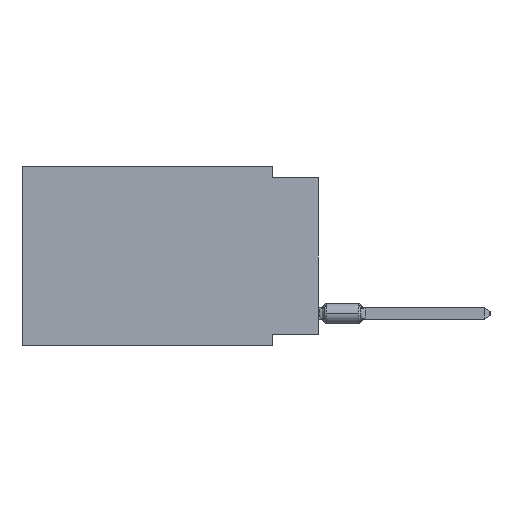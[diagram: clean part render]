
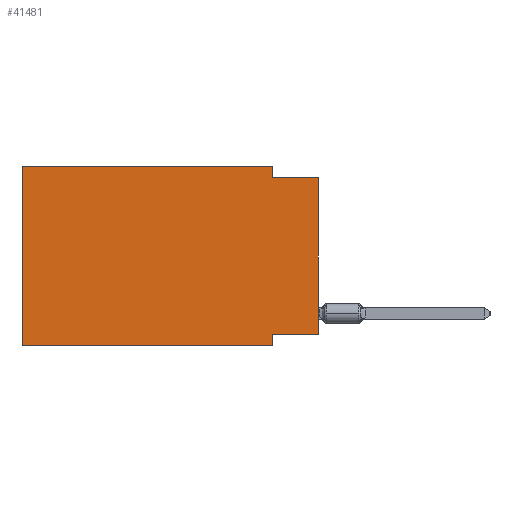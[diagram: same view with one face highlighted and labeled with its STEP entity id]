
A CAD part, left-side view. The second image highlights one B-rep face of the part: STEP entity #41481.
In plain terms, the highlighted planar face has unit normal (-1, 0, 0).
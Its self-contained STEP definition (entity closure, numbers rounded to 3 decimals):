
#156 = DIRECTION ( 'NONE',  ( 0., -1., 0. ) ) ;
#879 = VERTEX_POINT ( 'NONE', #2792 ) ;
#2080 = CARTESIAN_POINT ( 'NONE',  ( 0., 0., -0.635 ) ) ;
#2792 = CARTESIAN_POINT ( 'NONE',  ( 0., 2.54, -0.635 ) ) ;
#2931 = VECTOR ( 'NONE', #52530, 1000. ) ;
#3708 = DIRECTION ( 'NONE',  ( 0., 0., 1. ) ) ;
#5998 = LINE ( 'NONE', #48195, #9810 ) ;
#6533 = ORIENTED_EDGE ( 'NONE', *, *, #19204, .F. ) ;
#7318 = CARTESIAN_POINT ( 'NONE',  ( 0., 16.383, 0. ) ) ;
#8209 = EDGE_CURVE ( 'NONE', #28803, #879, #25545, .T. ) ;
#8283 = VECTOR ( 'NONE', #3708, 1000. ) ;
#8956 = VECTOR ( 'NONE', #33312, 1000. ) ;
#9810 = VECTOR ( 'NONE', #14686, 1000. ) ;
#10345 = EDGE_CURVE ( 'NONE', #23411, #52980, #48077, .T. ) ;
#10393 = EDGE_CURVE ( 'NONE', #23411, #51182, #37569, .T. ) ;
#11794 = DIRECTION ( 'NONE',  ( 1., 0., 0. ) ) ;
#12307 = ORIENTED_EDGE ( 'NONE', *, *, #23452, .F. ) ;
#14686 = DIRECTION ( 'NONE',  ( 0., -1., 0. ) ) ;
#15050 = LINE ( 'NONE', #23460, #21551 ) ;
#16343 = CARTESIAN_POINT ( 'NONE',  ( 0., 2.54, 0. ) ) ;
#18309 = VERTEX_POINT ( 'NONE', #25580 ) ;
#19204 = EDGE_CURVE ( 'NONE', #52980, #18309, #41939, .T. ) ;
#19668 = CARTESIAN_POINT ( 'NONE',  ( 0., 16.383, -9.906 ) ) ;
#21036 = PLANE ( 'NONE',  #47025 ) ;
#21551 = VECTOR ( 'NONE', #24274, 1000. ) ;
#23064 = EDGE_CURVE ( 'NONE', #35715, #18309, #45614, .T. ) ;
#23411 = VERTEX_POINT ( 'NONE', #28195 ) ;
#23452 = EDGE_CURVE ( 'NONE', #54804, #28803, #24275, .T. ) ;
#23460 = CARTESIAN_POINT ( 'NONE',  ( 0., 16.383, 0. ) ) ;
#23718 = EDGE_LOOP ( 'NONE', ( #28768, #26901, #28995, #12307, #45061, #27362, #6533, #38827 ) ) ;
#24274 = DIRECTION ( 'NONE',  ( 0., 0., 1. ) ) ;
#24275 = LINE ( 'NONE', #25092, #36502 ) ;
#24423 = DIRECTION ( 'NONE',  ( 0., 0., -1. ) ) ;
#24738 = CARTESIAN_POINT ( 'NONE',  ( 0., 2.54, 0. ) ) ;
#25092 = CARTESIAN_POINT ( 'NONE',  ( 0., 16.383, 0. ) ) ;
#25545 = LINE ( 'NONE', #16343, #41845 ) ;
#25580 = CARTESIAN_POINT ( 'NONE',  ( 0., 2.54, -9.906 ) ) ;
#26901 = ORIENTED_EDGE ( 'NONE', *, *, #37146, .F. ) ;
#27362 = ORIENTED_EDGE ( 'NONE', *, *, #23064, .T. ) ;
#28195 = CARTESIAN_POINT ( 'NONE',  ( 0., 0., -9.271 ) ) ;
#28768 = ORIENTED_EDGE ( 'NONE', *, *, #10393, .T. ) ;
#28803 = VERTEX_POINT ( 'NONE', #24738 ) ;
#28995 = ORIENTED_EDGE ( 'NONE', *, *, #8209, .F. ) ;
#32254 = DIRECTION ( 'NONE',  ( 0., -1., 0. ) ) ;
#32542 = CARTESIAN_POINT ( 'NONE',  ( 0., 2.54, -9.271 ) ) ;
#33312 = DIRECTION ( 'NONE',  ( 0., 0., -1. ) ) ;
#33832 = VECTOR ( 'NONE', #32254, 1000. ) ;
#35533 = CARTESIAN_POINT ( 'NONE',  ( 0., 0., -9.271 ) ) ;
#35715 = VERTEX_POINT ( 'NONE', #41806 ) ;
#36502 = VECTOR ( 'NONE', #156, 1000. ) ;
#37146 = EDGE_CURVE ( 'NONE', #879, #51182, #5998, .T. ) ;
#37477 = CARTESIAN_POINT ( 'NONE',  ( 0., 2.54, -9.906 ) ) ;
#37569 = LINE ( 'NONE', #54574, #8283 ) ;
#38827 = ORIENTED_EDGE ( 'NONE', *, *, #10345, .F. ) ;
#41481 = ADVANCED_FACE ( 'NONE', ( #45622 ), #21036, .F. ) ;
#41806 = CARTESIAN_POINT ( 'NONE',  ( 0., 16.383, -9.906 ) ) ;
#41845 = VECTOR ( 'NONE', #51202, 1000. ) ;
#41939 = LINE ( 'NONE', #37477, #8956 ) ;
#43421 = CARTESIAN_POINT ( 'NONE',  ( 0., 16.383, 0. ) ) ;
#45061 = ORIENTED_EDGE ( 'NONE', *, *, #47161, .F. ) ;
#45614 = LINE ( 'NONE', #19668, #33832 ) ;
#45622 = FACE_OUTER_BOUND ( 'NONE', #23718, .T. ) ;
#47025 = AXIS2_PLACEMENT_3D ( 'NONE', #7318, #11794, #24423 ) ;
#47161 = EDGE_CURVE ( 'NONE', #35715, #54804, #15050, .T. ) ;
#48077 = LINE ( 'NONE', #35533, #2931 ) ;
#48195 = CARTESIAN_POINT ( 'NONE',  ( 0., 0., -0.635 ) ) ;
#51182 = VERTEX_POINT ( 'NONE', #2080 ) ;
#51202 = DIRECTION ( 'NONE',  ( 0., 0., -1. ) ) ;
#52530 = DIRECTION ( 'NONE',  ( 0., 1., 0. ) ) ;
#52980 = VERTEX_POINT ( 'NONE', #32542 ) ;
#54574 = CARTESIAN_POINT ( 'NONE',  ( 0., 0., 0. ) ) ;
#54804 = VERTEX_POINT ( 'NONE', #43421 ) ;
